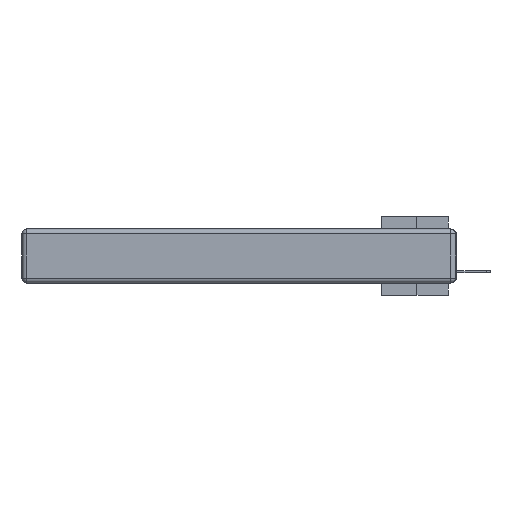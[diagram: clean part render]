
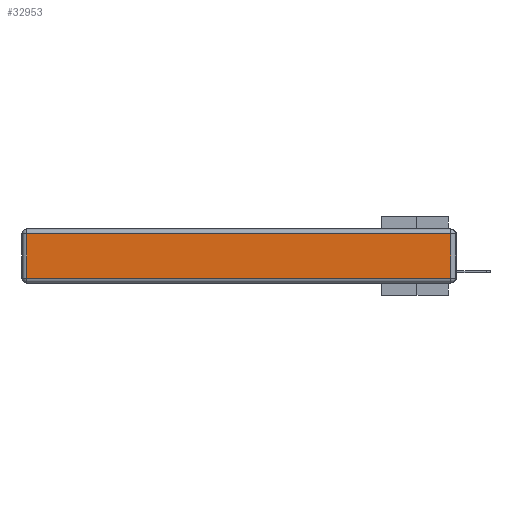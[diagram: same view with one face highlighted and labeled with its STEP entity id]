
A CAD part, left-side view. The second image highlights one B-rep face of the part: STEP entity #32953.
In plain terms, the highlighted planar face has unit normal (-1, 0, 0).
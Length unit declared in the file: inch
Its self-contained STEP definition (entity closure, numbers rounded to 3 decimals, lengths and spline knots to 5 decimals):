
#1567 = CARTESIAN_POINT ( 'NONE',  ( 0., 2.72, -0.343 ) ) ;
#3115 = CARTESIAN_POINT ( 'NONE',  ( 0., 0.03, -0.03 ) ) ;
#3370 = CARTESIAN_POINT ( 'NONE',  ( 0., 0., -0.343 ) ) ;
#3825 = EDGE_CURVE ( 'NONE', #19180, #11907, #14363, .T. ) ;
#4181 = VERTEX_POINT ( 'NONE', #35300 ) ;
#6058 = CARTESIAN_POINT ( 'NONE',  ( 0., 0., -0.313 ) ) ;
#6262 = DIRECTION ( 'NONE',  ( 0., -1., 0. ) ) ;
#7462 = VECTOR ( 'NONE', #6262, 39.37008 ) ;
#7753 = DIRECTION ( 'NONE',  ( 0., 0., -1. ) ) ;
#8691 = CARTESIAN_POINT ( 'NONE',  ( 0., 2.75, -0.03 ) ) ;
#9374 = DIRECTION ( 'NONE',  ( 0., 0., 1. ) ) ;
#9811 = CARTESIAN_POINT ( 'NONE',  ( 0., 2.72, -0.03 ) ) ;
#11698 = LINE ( 'NONE', #8691, #27889 ) ;
#11907 = VERTEX_POINT ( 'NONE', #38335 ) ;
#14363 = LINE ( 'NONE', #1567, #19060 ) ;
#15498 = DIRECTION ( 'NONE',  ( 0., 1., 0. ) ) ;
#15575 = PLANE ( 'NONE',  #35884 ) ;
#15980 = FACE_OUTER_BOUND ( 'NONE', #28450, .T. ) ;
#17101 = DIRECTION ( 'NONE',  ( 0., 0., 1. ) ) ;
#17358 = EDGE_CURVE ( 'NONE', #11907, #4181, #36451, .T. ) ;
#17630 = ORIENTED_EDGE ( 'NONE', *, *, #17358, .T. ) ;
#19060 = VECTOR ( 'NONE', #7753, 39.37008 ) ;
#19180 = VERTEX_POINT ( 'NONE', #9811 ) ;
#20028 = ORIENTED_EDGE ( 'NONE', *, *, #3825, .T. ) ;
#22083 = VECTOR ( 'NONE', #17101, 39.37008 ) ;
#22308 = LINE ( 'NONE', #22677, #22083 ) ;
#22677 = CARTESIAN_POINT ( 'NONE',  ( 0., 0.03, -0.343 ) ) ;
#25848 = EDGE_CURVE ( 'NONE', #30535, #19180, #11698, .T. ) ;
#27889 = VECTOR ( 'NONE', #15498, 39.37008 ) ;
#28313 = ORIENTED_EDGE ( 'NONE', *, *, #25848, .T. ) ;
#28450 = EDGE_LOOP ( 'NONE', ( #17630, #31581, #28313, #20028 ) ) ;
#30535 = VERTEX_POINT ( 'NONE', #3115 ) ;
#31581 = ORIENTED_EDGE ( 'NONE', *, *, #34512, .T. ) ;
#32953 = ADVANCED_FACE ( 'NONE', ( #15980 ), #15575, .T. ) ;
#33759 = DIRECTION ( 'NONE',  ( -1., 0., 0. ) ) ;
#34512 = EDGE_CURVE ( 'NONE', #4181, #30535, #22308, .T. ) ;
#35300 = CARTESIAN_POINT ( 'NONE',  ( 0., 0.03, -0.313 ) ) ;
#35884 = AXIS2_PLACEMENT_3D ( 'NONE', #3370, #33759, #9374 ) ;
#36451 = LINE ( 'NONE', #6058, #7462 ) ;
#38335 = CARTESIAN_POINT ( 'NONE',  ( 0., 2.72, -0.313 ) ) ;
